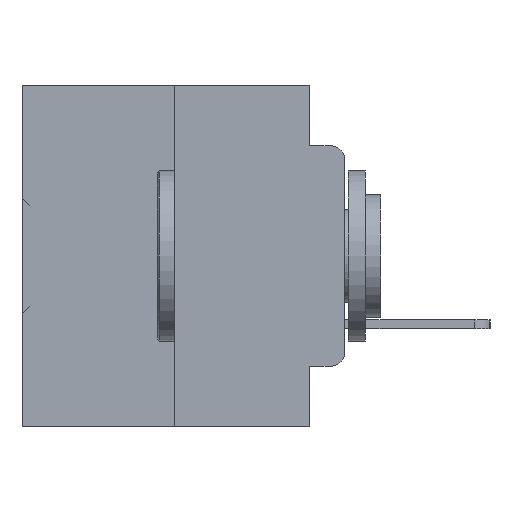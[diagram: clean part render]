
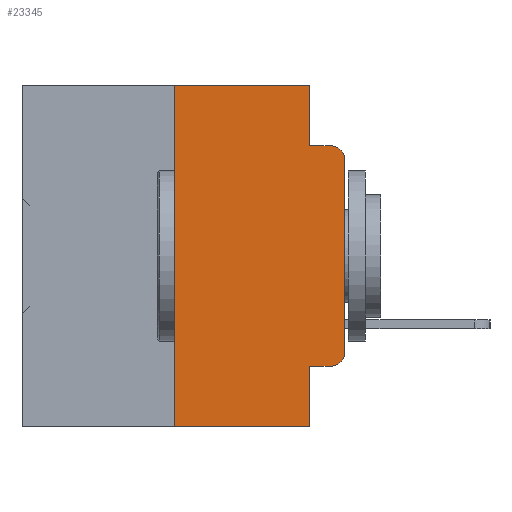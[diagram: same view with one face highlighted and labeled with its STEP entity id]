
A CAD part, left-side view. The second image highlights one B-rep face of the part: STEP entity #23345.
In plain terms, the highlighted planar face has unit normal (-1, 0, 0).
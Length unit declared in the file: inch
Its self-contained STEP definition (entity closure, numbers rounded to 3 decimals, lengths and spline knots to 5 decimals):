
#560 = VERTEX_POINT ( 'NONE', #19161 ) ;
#1030 = ORIENTED_EDGE ( 'NONE', *, *, #10471, .T. ) ;
#1626 = LINE ( 'NONE', #22831, #23795 ) ;
#1639 = VERTEX_POINT ( 'NONE', #24377 ) ;
#2377 = CARTESIAN_POINT ( 'NONE',  ( 0., 0.02, -0.3915 ) ) ;
#2675 = EDGE_CURVE ( 'NONE', #10641, #560, #16585, .T. ) ;
#2888 = VERTEX_POINT ( 'NONE', #27091 ) ;
#4653 = EDGE_CURVE ( 'NONE', #560, #14569, #9218, .T. ) ;
#5177 = CARTESIAN_POINT ( 'NONE',  ( 0., 0.473, 0. ) ) ;
#5188 = CARTESIAN_POINT ( 'NONE',  ( 0., 0.02, -0.1085 ) ) ;
#5324 = DIRECTION ( 'NONE',  ( 0., 0., -1. ) ) ;
#5729 = CIRCLE ( 'NONE', #17629, 0.02 ) ;
#6416 = DIRECTION ( 'NONE',  ( 0., -1., 0. ) ) ;
#6788 = LINE ( 'NONE', #23913, #27102 ) ;
#6956 = LINE ( 'NONE', #22617, #35900 ) ;
#8073 = DIRECTION ( 'NONE',  ( 0., 0., -1. ) ) ;
#8088 = DIRECTION ( 'NONE',  ( 0., 0., -1. ) ) ;
#8523 = EDGE_CURVE ( 'NONE', #1639, #14569, #5729, .T. ) ;
#9218 = LINE ( 'NONE', #26600, #31375 ) ;
#9301 = VECTOR ( 'NONE', #28028, 39.37008 ) ;
#10411 = CARTESIAN_POINT ( 'NONE',  ( 0., 0.02, -0.0885 ) ) ;
#10471 = EDGE_CURVE ( 'NONE', #13453, #1639, #1626, .T. ) ;
#10618 = ORIENTED_EDGE ( 'NONE', *, *, #4653, .F. ) ;
#10641 = VERTEX_POINT ( 'NONE', #23605 ) ;
#10719 = CARTESIAN_POINT ( 'NONE',  ( 0., 0., -0.3915 ) ) ;
#11994 = LINE ( 'NONE', #25079, #9301 ) ;
#12045 = VECTOR ( 'NONE', #18555, 39.37008 ) ;
#13453 = VERTEX_POINT ( 'NONE', #10719 ) ;
#14191 = ORIENTED_EDGE ( 'NONE', *, *, #32516, .F. ) ;
#14569 = VERTEX_POINT ( 'NONE', #10411 ) ;
#14667 = DIRECTION ( 'NONE',  ( 0., -1., 0. ) ) ;
#14904 = AXIS2_PLACEMENT_3D ( 'NONE', #5177, #25356, #8073 ) ;
#16397 = ORIENTED_EDGE ( 'NONE', *, *, #8523, .T. ) ;
#16585 = LINE ( 'NONE', #29148, #23415 ) ;
#16667 = EDGE_CURVE ( 'NONE', #28334, #2888, #6788, .T. ) ;
#16847 = CARTESIAN_POINT ( 'NONE',  ( 0., 0.25, 0. ) ) ;
#17629 = AXIS2_PLACEMENT_3D ( 'NONE', #5188, #25372, #8088 ) ;
#17672 = CIRCLE ( 'NONE', #22339, 0.02 ) ;
#17673 = CARTESIAN_POINT ( 'NONE',  ( 0., 0.02, -0.4115 ) ) ;
#17838 = LINE ( 'NONE', #34990, #24662 ) ;
#18555 = DIRECTION ( 'NONE',  ( 0., -1., 0. ) ) ;
#19161 = CARTESIAN_POINT ( 'NONE',  ( 0., 0.051, -0.0885 ) ) ;
#19929 = DIRECTION ( 'NONE',  ( 0., 0., 1. ) ) ;
#20962 = ORIENTED_EDGE ( 'NONE', *, *, #30124, .F. ) ;
#22339 = AXIS2_PLACEMENT_3D ( 'NONE', #2377, #22568, #5324 ) ;
#22404 = PLANE ( 'NONE',  #14904 ) ;
#22436 = VERTEX_POINT ( 'NONE', #26421 ) ;
#22568 = DIRECTION ( 'NONE',  ( -1., 0., 0. ) ) ;
#22617 = CARTESIAN_POINT ( 'NONE',  ( 0., 0.25, 0. ) ) ;
#22716 = EDGE_CURVE ( 'NONE', #26483, #13453, #17672, .T. ) ;
#22739 = VERTEX_POINT ( 'NONE', #16847 ) ;
#22831 = CARTESIAN_POINT ( 'NONE',  ( 0., 0., 0. ) ) ;
#23345 = ADVANCED_FACE ( 'NONE', ( #34455 ), #22404, .F. ) ;
#23415 = VECTOR ( 'NONE', #32069, 39.37008 ) ;
#23605 = CARTESIAN_POINT ( 'NONE',  ( 0., 0.051, 0. ) ) ;
#23795 = VECTOR ( 'NONE', #19929, 39.37008 ) ;
#23913 = CARTESIAN_POINT ( 'NONE',  ( 0., 0.473, -0.5 ) ) ;
#24267 = CARTESIAN_POINT ( 'NONE',  ( 0., 0.051, -0.4115 ) ) ;
#24377 = CARTESIAN_POINT ( 'NONE',  ( 0., 0., -0.1085 ) ) ;
#24617 = ORIENTED_EDGE ( 'NONE', *, *, #30572, .F. ) ;
#24662 = VECTOR ( 'NONE', #14667, 39.37008 ) ;
#25079 = CARTESIAN_POINT ( 'NONE',  ( 0., 0.051, 0. ) ) ;
#25356 = DIRECTION ( 'NONE',  ( 1., 0., 0. ) ) ;
#25372 = DIRECTION ( 'NONE',  ( -1., 0., 0. ) ) ;
#25564 = DIRECTION ( 'NONE',  ( 0., 0., 1. ) ) ;
#26421 = CARTESIAN_POINT ( 'NONE',  ( 0., 0.051, -0.4115 ) ) ;
#26446 = ORIENTED_EDGE ( 'NONE', *, *, #26661, .T. ) ;
#26483 = VERTEX_POINT ( 'NONE', #17673 ) ;
#26600 = CARTESIAN_POINT ( 'NONE',  ( 0., 0.051, -0.0885 ) ) ;
#26661 = EDGE_CURVE ( 'NONE', #22436, #26483, #35159, .T. ) ;
#26835 = DIRECTION ( 'NONE',  ( 0., -1., 0. ) ) ;
#27091 = CARTESIAN_POINT ( 'NONE',  ( 0., 0.051, -0.5 ) ) ;
#27102 = VECTOR ( 'NONE', #26835, 39.37008 ) ;
#28028 = DIRECTION ( 'NONE',  ( 0., 0., -1. ) ) ;
#28334 = VERTEX_POINT ( 'NONE', #29791 ) ;
#29148 = CARTESIAN_POINT ( 'NONE',  ( 0., 0.051, 0. ) ) ;
#29645 = ORIENTED_EDGE ( 'NONE', *, *, #16667, .T. ) ;
#29791 = CARTESIAN_POINT ( 'NONE',  ( 0., 0.25, -0.5 ) ) ;
#30124 = EDGE_CURVE ( 'NONE', #22739, #10641, #17838, .T. ) ;
#30572 = EDGE_CURVE ( 'NONE', #22436, #2888, #11994, .T. ) ;
#31375 = VECTOR ( 'NONE', #6416, 39.37008 ) ;
#31942 = EDGE_LOOP ( 'NONE', ( #1030, #16397, #10618, #34617, #20962, #14191, #29645, #24617, #26446, #34177 ) ) ;
#32069 = DIRECTION ( 'NONE',  ( 0., 0., -1. ) ) ;
#32516 = EDGE_CURVE ( 'NONE', #28334, #22739, #6956, .T. ) ;
#34177 = ORIENTED_EDGE ( 'NONE', *, *, #22716, .T. ) ;
#34455 = FACE_OUTER_BOUND ( 'NONE', #31942, .T. ) ;
#34617 = ORIENTED_EDGE ( 'NONE', *, *, #2675, .F. ) ;
#34990 = CARTESIAN_POINT ( 'NONE',  ( 0., 0.473, 0. ) ) ;
#35159 = LINE ( 'NONE', #24267, #12045 ) ;
#35900 = VECTOR ( 'NONE', #25564, 39.37008 ) ;
